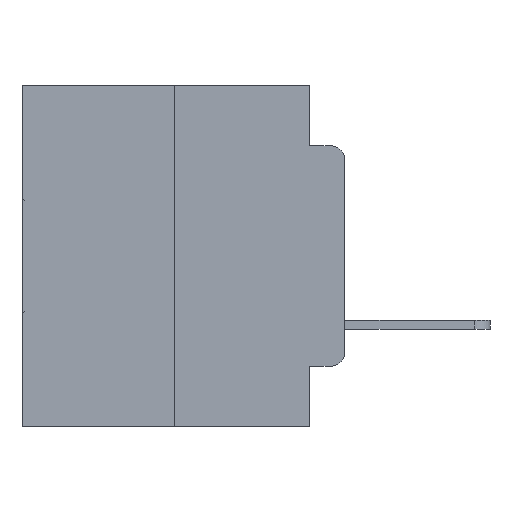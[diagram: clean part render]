
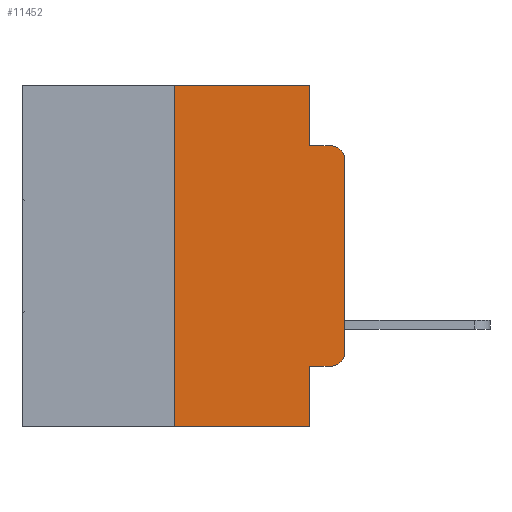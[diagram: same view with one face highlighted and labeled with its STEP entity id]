
A CAD part, left-side view. The second image highlights one B-rep face of the part: STEP entity #11452.
In plain terms, the highlighted planar face has unit normal (-1, 0, 0).
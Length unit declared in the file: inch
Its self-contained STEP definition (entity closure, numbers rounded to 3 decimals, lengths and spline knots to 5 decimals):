
#46 = DIRECTION ( 'NONE',  ( 1., 0., 0. ) ) ;
#58 = ORIENTED_EDGE ( 'NONE', *, *, #18770, .F. ) ;
#103 = CARTESIAN_POINT ( 'NONE',  ( 0., 0.02, -0.1085 ) ) ;
#826 = CARTESIAN_POINT ( 'NONE',  ( 0., 0., 0. ) ) ;
#1488 = ORIENTED_EDGE ( 'NONE', *, *, #18996, .T. ) ;
#1789 = ORIENTED_EDGE ( 'NONE', *, *, #20131, .T. ) ;
#2389 = LINE ( 'NONE', #20910, #25830 ) ;
#2689 = DIRECTION ( 'NONE',  ( -1., 0., 0. ) ) ;
#2904 = DIRECTION ( 'NONE',  ( 0., 0., -1. ) ) ;
#3252 = LINE ( 'NONE', #20301, #16668 ) ;
#3595 = CARTESIAN_POINT ( 'NONE',  ( 0., 0.051, -0.0885 ) ) ;
#3983 = EDGE_LOOP ( 'NONE', ( #25226, #26342, #26803, #26907, #27192, #28012, #1789, #58, #1488, #14362 ) ) ;
#4103 = CARTESIAN_POINT ( 'NONE',  ( 0., 0.051, 0. ) ) ;
#4627 = CARTESIAN_POINT ( 'NONE',  ( 0., 0., -0.1085 ) ) ;
#6024 = CIRCLE ( 'NONE', #23357, 0.02 ) ;
#6096 = DIRECTION ( 'NONE',  ( 0., -1., 0. ) ) ;
#6778 = CARTESIAN_POINT ( 'NONE',  ( 0., 0.051, -0.5 ) ) ;
#7339 = DIRECTION ( 'NONE',  ( 0., 0., 1. ) ) ;
#7774 = DIRECTION ( 'NONE',  ( 0., -1., 0. ) ) ;
#8552 = CARTESIAN_POINT ( 'NONE',  ( 0., 0.051, -0.4115 ) ) ;
#8623 = CARTESIAN_POINT ( 'NONE',  ( 0., 0., -0.3915 ) ) ;
#9095 = CARTESIAN_POINT ( 'NONE',  ( 0., 0.473, -0.5 ) ) ;
#9283 = EDGE_CURVE ( 'NONE', #27598, #19235, #3252, .T. ) ;
#9304 = CARTESIAN_POINT ( 'NONE',  ( 0., 0.02, -0.0885 ) ) ;
#9923 = VERTEX_POINT ( 'NONE', #4627 ) ;
#10245 = VECTOR ( 'NONE', #6096, 39.37008 ) ;
#10995 = VECTOR ( 'NONE', #27865, 39.37008 ) ;
#11452 = ADVANCED_FACE ( 'NONE', ( #26865 ), #12617, .F. ) ;
#12617 = PLANE ( 'NONE',  #23831 ) ;
#13759 = DIRECTION ( 'NONE',  ( 0., -1., 0. ) ) ;
#14362 = ORIENTED_EDGE ( 'NONE', *, *, #18961, .T. ) ;
#15329 = VERTEX_POINT ( 'NONE', #8623 ) ;
#15439 = CARTESIAN_POINT ( 'NONE',  ( 0., 0.02, -0.4115 ) ) ;
#16668 = VECTOR ( 'NONE', #20264, 39.37008 ) ;
#17034 = CARTESIAN_POINT ( 'NONE',  ( 0., 0.02, -0.3915 ) ) ;
#17156 = DIRECTION ( 'NONE',  ( 0., 0., -1. ) ) ;
#17196 = DIRECTION ( 'NONE',  ( -1., 0., 0. ) ) ;
#17398 = VERTEX_POINT ( 'NONE', #8552 ) ;
#18087 = LINE ( 'NONE', #20532, #28184 ) ;
#18563 = EDGE_CURVE ( 'NONE', #25721, #27598, #19722, .T. ) ;
#18571 = EDGE_CURVE ( 'NONE', #19235, #23529, #27309, .T. ) ;
#18770 = EDGE_CURVE ( 'NONE', #17398, #28921, #18087, .T. ) ;
#18876 = EDGE_CURVE ( 'NONE', #22181, #25721, #2389, .T. ) ;
#18961 = EDGE_CURVE ( 'NONE', #24774, #15329, #6024, .T. ) ;
#18987 = LINE ( 'NONE', #826, #28931 ) ;
#18996 = EDGE_CURVE ( 'NONE', #17398, #24774, #28436, .T. ) ;
#19189 = DIRECTION ( 'NONE',  ( 0., 0., -1. ) ) ;
#19235 = VERTEX_POINT ( 'NONE', #19805 ) ;
#19674 = LINE ( 'NONE', #9095, #23905 ) ;
#19722 = LINE ( 'NONE', #23859, #10995 ) ;
#19756 = EDGE_CURVE ( 'NONE', #9923, #23529, #22321, .T. ) ;
#19805 = CARTESIAN_POINT ( 'NONE',  ( 0., 0.051, -0.0885 ) ) ;
#20131 = EDGE_CURVE ( 'NONE', #22181, #28921, #19674, .T. ) ;
#20264 = DIRECTION ( 'NONE',  ( 0., 0., -1. ) ) ;
#20301 = CARTESIAN_POINT ( 'NONE',  ( 0., 0.051, 0. ) ) ;
#20532 = CARTESIAN_POINT ( 'NONE',  ( 0., 0.051, 0. ) ) ;
#20910 = CARTESIAN_POINT ( 'NONE',  ( 0., 0.25, 0. ) ) ;
#22181 = VERTEX_POINT ( 'NONE', #24979 ) ;
#22321 = CIRCLE ( 'NONE', #26852, 0.02 ) ;
#22693 = DIRECTION ( 'NONE',  ( 0., 0., -1. ) ) ;
#23276 = VECTOR ( 'NONE', #7774, 39.37008 ) ;
#23357 = AXIS2_PLACEMENT_3D ( 'NONE', #17034, #2689, #19189 ) ;
#23529 = VERTEX_POINT ( 'NONE', #9304 ) ;
#23831 = AXIS2_PLACEMENT_3D ( 'NONE', #27349, #46, #17156 ) ;
#23859 = CARTESIAN_POINT ( 'NONE',  ( 0., 0.473, 0. ) ) ;
#23905 = VECTOR ( 'NONE', #13759, 39.37008 ) ;
#24124 = CARTESIAN_POINT ( 'NONE',  ( 0., 0.25, 0. ) ) ;
#24774 = VERTEX_POINT ( 'NONE', #15439 ) ;
#24979 = CARTESIAN_POINT ( 'NONE',  ( 0., 0.25, -0.5 ) ) ;
#25226 = ORIENTED_EDGE ( 'NONE', *, *, #26420, .T. ) ;
#25721 = VERTEX_POINT ( 'NONE', #24124 ) ;
#25830 = VECTOR ( 'NONE', #7339, 39.37008 ) ;
#26342 = ORIENTED_EDGE ( 'NONE', *, *, #19756, .T. ) ;
#26420 = EDGE_CURVE ( 'NONE', #15329, #9923, #18987, .T. ) ;
#26803 = ORIENTED_EDGE ( 'NONE', *, *, #18571, .F. ) ;
#26852 = AXIS2_PLACEMENT_3D ( 'NONE', #103, #17196, #2904 ) ;
#26865 = FACE_OUTER_BOUND ( 'NONE', #3983, .T. ) ;
#26907 = ORIENTED_EDGE ( 'NONE', *, *, #9283, .F. ) ;
#27192 = ORIENTED_EDGE ( 'NONE', *, *, #18563, .F. ) ;
#27309 = LINE ( 'NONE', #3595, #10245 ) ;
#27349 = CARTESIAN_POINT ( 'NONE',  ( 0., 0.473, 0. ) ) ;
#27598 = VERTEX_POINT ( 'NONE', #4103 ) ;
#27865 = DIRECTION ( 'NONE',  ( 0., -1., 0. ) ) ;
#27870 = DIRECTION ( 'NONE',  ( 0., 0., 1. ) ) ;
#28012 = ORIENTED_EDGE ( 'NONE', *, *, #18876, .F. ) ;
#28184 = VECTOR ( 'NONE', #22693, 39.37008 ) ;
#28436 = LINE ( 'NONE', #29049, #23276 ) ;
#28921 = VERTEX_POINT ( 'NONE', #6778 ) ;
#28931 = VECTOR ( 'NONE', #27870, 39.37008 ) ;
#29049 = CARTESIAN_POINT ( 'NONE',  ( 0., 0.051, -0.4115 ) ) ;
